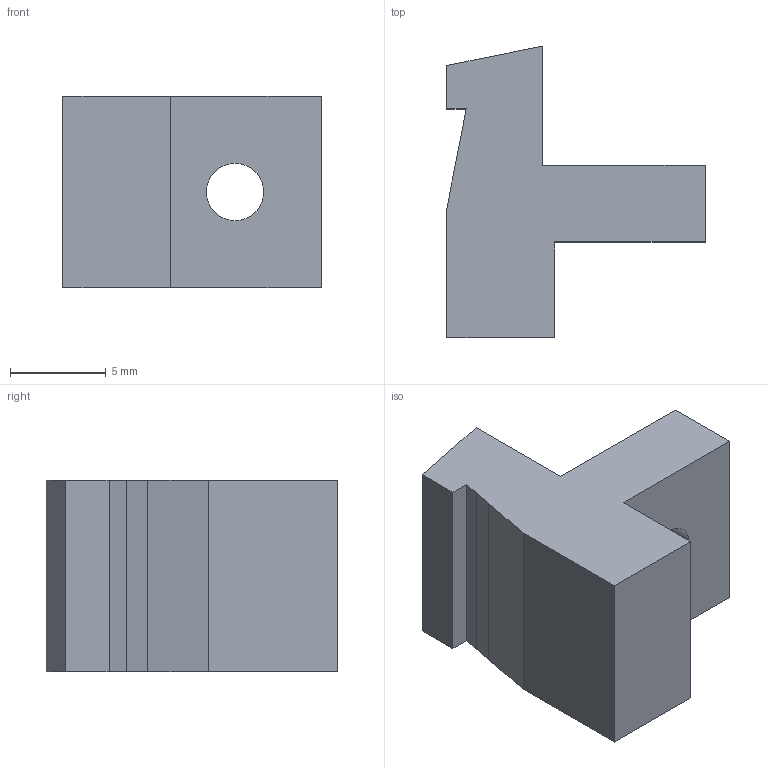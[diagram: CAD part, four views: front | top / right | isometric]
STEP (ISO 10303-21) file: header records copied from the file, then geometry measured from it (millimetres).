
FILE_DESCRIPTION (( 'STEP AP203' ), '1' );
FILE_NAME ('MOD9_V3_Feed_Ramp.STEP', '2020-12-23T17:52:51', ( '' ), ( '' ), 'SwSTEP 2.0', 'SolidWorks 2019', '' );
FILE_SCHEMA (( 'CONFIG_CONTROL_DESIGN' ));
Length unit declared in the file: millimetre
Products named in the file (1): MOD9_V3_Feed_Ramp
Bounding box: 13.5 x 15.24 x 10 mm (x, y, z)
Volume: 1026.5 mm3; surface area: 810.9 mm2
Topology: 1 solids, 1 shells, 20 faces, 52 edges, 34 vertices
Faces by surface type: plane 16, cylinder 2, cone 2
Entity records: 687 total; most frequent: CARTESIAN_POINT 107, ORIENTED_EDGE 104, DIRECTION 100, EDGE_CURVE 52, LINE 46, VECTOR 46, VERTEX_POINT 34, AXIS2_PLACEMENT_3D 27
